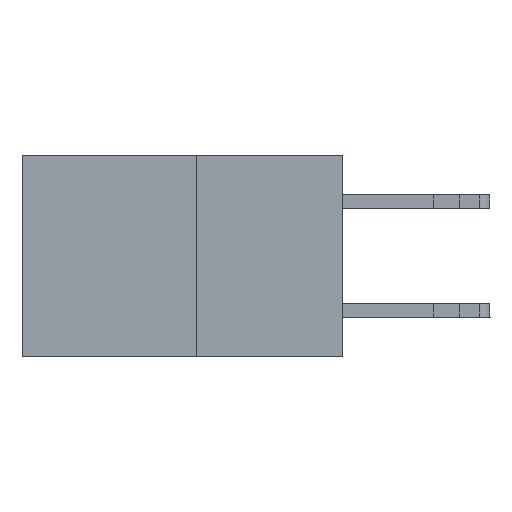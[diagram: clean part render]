
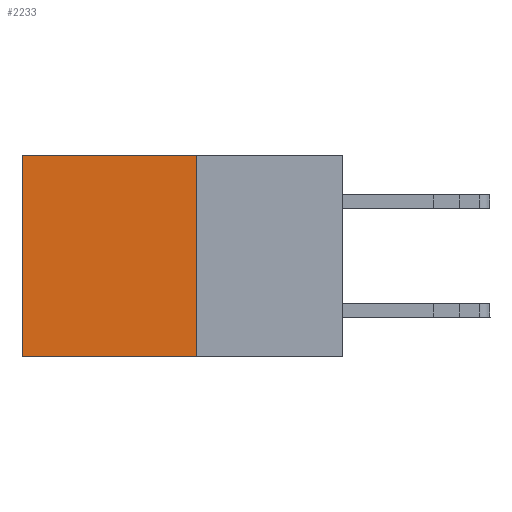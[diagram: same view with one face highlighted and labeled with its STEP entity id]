
A CAD part, left-side view. The second image highlights one B-rep face of the part: STEP entity #2233.
In plain terms, the highlighted planar face has unit normal (-1, 0, 0).
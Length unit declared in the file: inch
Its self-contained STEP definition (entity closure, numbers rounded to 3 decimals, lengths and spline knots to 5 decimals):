
#1547 = CARTESIAN_POINT ( 'NONE',  ( 0.277, 0.27, -0.37 ) ) ;
#1551 = AXIS2_PLACEMENT_3D ( 'NONE', #5891, #4804, #4900 ) ;
#1894 = EDGE_CURVE ( 'NONE', #7342, #22240, #18719, .T. ) ;
#2233 = ADVANCED_FACE ( 'NONE', ( #11236 ), #5500, .F. ) ;
#2370 = VECTOR ( 'NONE', #12900, 39.37008 ) ;
#2538 = CARTESIAN_POINT ( 'NONE',  ( 0.277, 0.27, -0.37 ) ) ;
#4186 = CARTESIAN_POINT ( 'NONE',  ( 0.277, 0.59, -0.37 ) ) ;
#4326 = VECTOR ( 'NONE', #11679, 39.37008 ) ;
#4804 = DIRECTION ( 'NONE',  ( 1., 0., 0. ) ) ;
#4900 = DIRECTION ( 'NONE',  ( 0., 0., -1. ) ) ;
#5500 = PLANE ( 'NONE',  #1551 ) ;
#5891 = CARTESIAN_POINT ( 'NONE',  ( 0.277, 0.27, -0.37 ) ) ;
#6508 = CARTESIAN_POINT ( 'NONE',  ( 0.277, 0.27, 0. ) ) ;
#6746 = ORIENTED_EDGE ( 'NONE', *, *, #13548, .T. ) ;
#6985 = EDGE_CURVE ( 'NONE', #10532, #9366, #8943, .T. ) ;
#7000 = LINE ( 'NONE', #4186, #2370 ) ;
#7342 = VERTEX_POINT ( 'NONE', #2538 ) ;
#8943 = LINE ( 'NONE', #6508, #4326 ) ;
#9366 = VERTEX_POINT ( 'NONE', #9972 ) ;
#9623 = VECTOR ( 'NONE', #15819, 39.37008 ) ;
#9842 = ORIENTED_EDGE ( 'NONE', *, *, #6985, .T. ) ;
#9972 = CARTESIAN_POINT ( 'NONE',  ( 0.277, 0.59, 0. ) ) ;
#10419 = EDGE_LOOP ( 'NONE', ( #6746, #16274, #20936, #9842 ) ) ;
#10532 = VERTEX_POINT ( 'NONE', #21407 ) ;
#11236 = FACE_OUTER_BOUND ( 'NONE', #10419, .T. ) ;
#11679 = DIRECTION ( 'NONE',  ( 0., 1., 0. ) ) ;
#12900 = DIRECTION ( 'NONE',  ( 0., 0., -1. ) ) ;
#13548 = EDGE_CURVE ( 'NONE', #9366, #22240, #7000, .T. ) ;
#13710 = CARTESIAN_POINT ( 'NONE',  ( 0.277, 0.59, -0.37 ) ) ;
#14017 = EDGE_CURVE ( 'NONE', #10532, #7342, #16145, .T. ) ;
#15411 = DIRECTION ( 'NONE',  ( 0., 0., -1. ) ) ;
#15727 = CARTESIAN_POINT ( 'NONE',  ( 0.277, 0.27, -0.37 ) ) ;
#15819 = DIRECTION ( 'NONE',  ( 0., 1., 0. ) ) ;
#16145 = LINE ( 'NONE', #1547, #19621 ) ;
#16274 = ORIENTED_EDGE ( 'NONE', *, *, #1894, .F. ) ;
#18719 = LINE ( 'NONE', #15727, #9623 ) ;
#19621 = VECTOR ( 'NONE', #15411, 39.37008 ) ;
#20936 = ORIENTED_EDGE ( 'NONE', *, *, #14017, .F. ) ;
#21407 = CARTESIAN_POINT ( 'NONE',  ( 0.277, 0.27, 0. ) ) ;
#22240 = VERTEX_POINT ( 'NONE', #13710 ) ;
